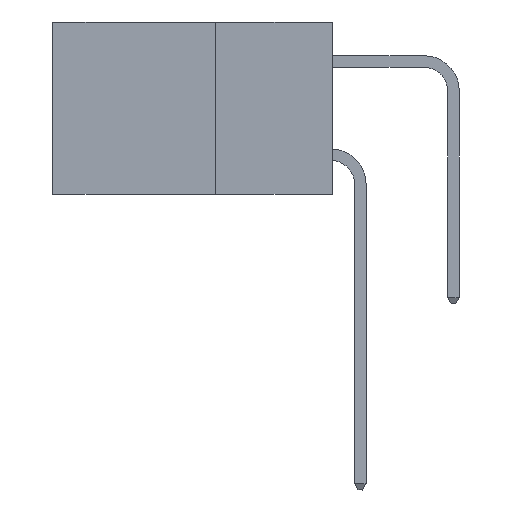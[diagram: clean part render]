
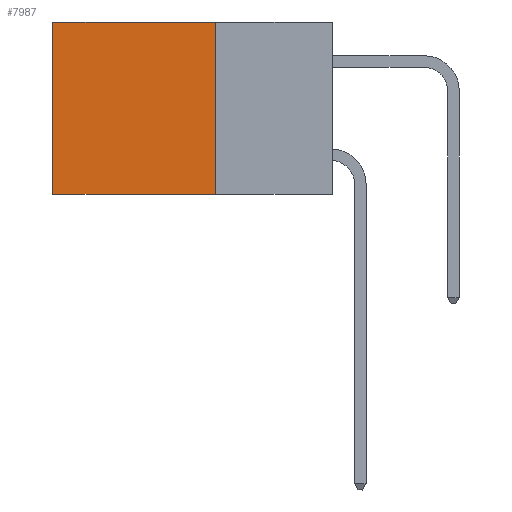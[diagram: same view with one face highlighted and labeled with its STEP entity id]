
A CAD part, left-side view. The second image highlights one B-rep face of the part: STEP entity #7987.
In plain terms, the highlighted planar face has unit normal (-1, 0, 0).
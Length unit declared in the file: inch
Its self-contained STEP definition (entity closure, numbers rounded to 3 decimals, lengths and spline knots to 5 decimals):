
#368 = LINE ( 'NONE', #7653, #10760 ) ;
#565 = DIRECTION ( 'NONE',  ( 0., 1., 0. ) ) ;
#1213 = CARTESIAN_POINT ( 'NONE',  ( 0.2615, 0.25, 0. ) ) ;
#1324 = CARTESIAN_POINT ( 'NONE',  ( 0.2615, 0.25, -0.37 ) ) ;
#2496 = EDGE_CURVE ( 'NONE', #10213, #6971, #3699, .T. ) ;
#3344 = EDGE_CURVE ( 'NONE', #10213, #15536, #368, .T. ) ;
#3572 = CARTESIAN_POINT ( 'NONE',  ( 0.2615, 0.6, -0.37 ) ) ;
#3699 = LINE ( 'NONE', #9643, #14246 ) ;
#3838 = CARTESIAN_POINT ( 'NONE',  ( 0.2615, 0.25, -0.37 ) ) ;
#4380 = EDGE_LOOP ( 'NONE', ( #9986, #12767, #10487, #9761 ) ) ;
#4904 = DIRECTION ( 'NONE',  ( 1., 0., 0. ) ) ;
#5132 = PLANE ( 'NONE',  #5255 ) ;
#5255 = AXIS2_PLACEMENT_3D ( 'NONE', #3838, #4904, #7257 ) ;
#5454 = EDGE_CURVE ( 'NONE', #6971, #14239, #13770, .T. ) ;
#5579 = CARTESIAN_POINT ( 'NONE',  ( 0.2615, 0.25, -0.37 ) ) ;
#6018 = DIRECTION ( 'NONE',  ( 0., 1., 0. ) ) ;
#6466 = CARTESIAN_POINT ( 'NONE',  ( 0.2615, 0.6, 0. ) ) ;
#6524 = DIRECTION ( 'NONE',  ( 0., 0., -1. ) ) ;
#6971 = VERTEX_POINT ( 'NONE', #6466 ) ;
#7257 = DIRECTION ( 'NONE',  ( 0., 0., -1. ) ) ;
#7653 = CARTESIAN_POINT ( 'NONE',  ( 0.2615, 0.25, -0.37 ) ) ;
#7987 = ADVANCED_FACE ( 'NONE', ( #15404 ), #5132, .F. ) ;
#8830 = VECTOR ( 'NONE', #565, 39.37008 ) ;
#9643 = CARTESIAN_POINT ( 'NONE',  ( 0.2615, 0.25, 0. ) ) ;
#9761 = ORIENTED_EDGE ( 'NONE', *, *, #2496, .T. ) ;
#9954 = EDGE_CURVE ( 'NONE', #15536, #14239, #13839, .T. ) ;
#9986 = ORIENTED_EDGE ( 'NONE', *, *, #5454, .T. ) ;
#10068 = CARTESIAN_POINT ( 'NONE',  ( 0.2615, 0.6, -0.37 ) ) ;
#10213 = VERTEX_POINT ( 'NONE', #1213 ) ;
#10258 = DIRECTION ( 'NONE',  ( 0., 0., -1. ) ) ;
#10487 = ORIENTED_EDGE ( 'NONE', *, *, #3344, .F. ) ;
#10760 = VECTOR ( 'NONE', #10258, 39.37008 ) ;
#11099 = VECTOR ( 'NONE', #6524, 39.37008 ) ;
#12767 = ORIENTED_EDGE ( 'NONE', *, *, #9954, .F. ) ;
#13770 = LINE ( 'NONE', #10068, #11099 ) ;
#13839 = LINE ( 'NONE', #5579, #8830 ) ;
#14239 = VERTEX_POINT ( 'NONE', #3572 ) ;
#14246 = VECTOR ( 'NONE', #6018, 39.37008 ) ;
#15404 = FACE_OUTER_BOUND ( 'NONE', #4380, .T. ) ;
#15536 = VERTEX_POINT ( 'NONE', #1324 ) ;
